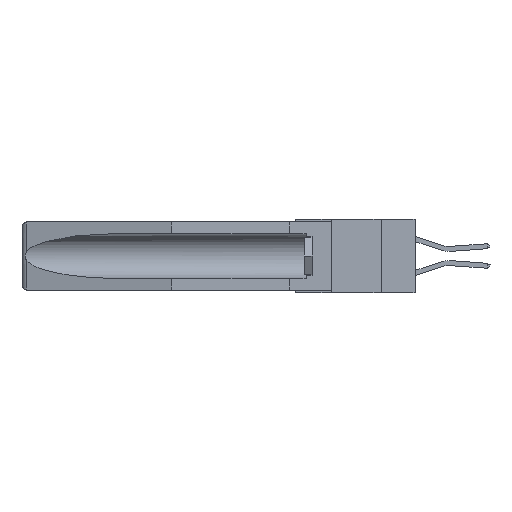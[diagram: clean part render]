
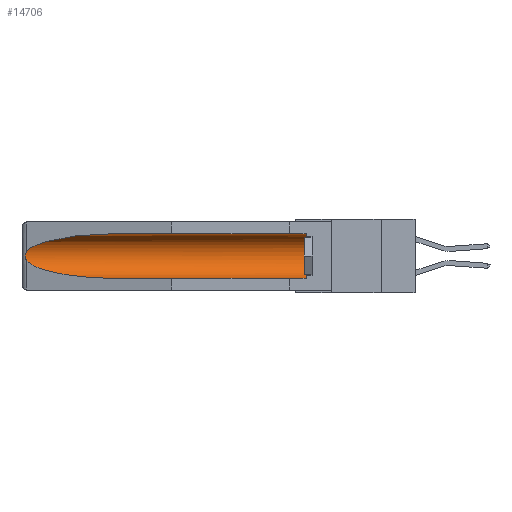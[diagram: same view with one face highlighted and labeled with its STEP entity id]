
A CAD part, left-side view. The second image highlights one B-rep face of the part: STEP entity #14706.
In plain terms, the highlighted cylindrical face has radius 2.857 mm (diameter 5.715 mm), a partial arc.
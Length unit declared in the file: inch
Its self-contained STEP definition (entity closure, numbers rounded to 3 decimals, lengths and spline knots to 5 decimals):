
#239 = DIRECTION ( 'NONE',  ( 0., 0., 1. ) ) ;
#935 = DIRECTION ( 'NONE',  ( 0., 1., 0. ) ) ;
#995 = VECTOR ( 'NONE', #17633, 39.37008 ) ;
#1039 = EDGE_CURVE ( 'NONE', #2040, #2214, #3369, .T. ) ;
#1953 = CARTESIAN_POINT ( 'NONE',  ( 0.26654, 1.53092, -0.15636 ) ) ;
#2040 = VERTEX_POINT ( 'NONE', #22768 ) ;
#2155 = CARTESIAN_POINT ( 'NONE',  ( 0.2673, 1.53269, -0.17917 ) ) ;
#2214 = VERTEX_POINT ( 'NONE', #13699 ) ;
#2488 = LINE ( 'NONE', #27379, #21067 ) ;
#3369 = B_SPLINE_CURVE_WITH_KNOTS ( 'NONE', 3,
 ( #18769, #9451, #1953, #23361, #26036, #16566, #2155, #11779, #23762, #25623 ),
 .UNSPECIFIED., .F., .F.,
 ( 4, 2, 2, 2, 4 ),
 ( 0., 0.00029, 0.00058, 0.00087, 0.00117 ),
 .UNSPECIFIED. ) ;
#3976 = VERTEX_POINT ( 'NONE', #26563 ) ;
#4784 = ORIENTED_EDGE ( 'NONE', *, *, #29915, .T. ) ;
#5179 = CARTESIAN_POINT ( 'NONE',  ( 0.21114, 1.30732, -0.059 ) ) ;
#5483 = CARTESIAN_POINT ( 'NONE',  ( 0.26537, 1.52718, -0.14972 ) ) ;
#5624 = AXIS2_PLACEMENT_3D ( 'NONE', #7690, #24319, #239 ) ;
#6420 = VERTEX_POINT ( 'NONE', #10971 ) ;
#7472 = CARTESIAN_POINT ( 'NONE',  ( 0.155, 1.07973, -0.059 ) ) ;
#7690 = CARTESIAN_POINT ( 'NONE',  ( 0.155, -0.30754, -0.1715 ) ) ;
#8312 = CARTESIAN_POINT ( 'NONE',  ( 0.155, -0.30754, -0.284 ) ) ;
#8531 = CARTESIAN_POINT ( 'NONE',  ( 0.26537, 1.52718, -0.19328 ) ) ;
#8636 = CARTESIAN_POINT ( 'NONE',  ( 0.21114, 1.30732, -0.284 ) ) ;
#9451 = CARTESIAN_POINT ( 'NONE',  ( 0.26597, 1.52961, -0.15275 ) ) ;
#9853 = ORIENTED_EDGE ( 'NONE', *, *, #19906, .F. ) ;
#9854 =( BOUNDED_CURVE ( )  B_SPLINE_CURVE ( 3, ( #8531, #11002, #8636, #13080 ),
 .UNSPECIFIED., .F., .F. ) 
 B_SPLINE_CURVE_WITH_KNOTS ( ( 4, 4 ),
 ( 0.1948, 1.5708 ),
 .UNSPECIFIED. ) 
 CURVE ( )  GEOMETRIC_REPRESENTATION_ITEM ( )  RATIONAL_B_SPLINE_CURVE ( ( 1., 0.848, 0.848, 1. ) ) 
 REPRESENTATION_ITEM ( '' )  );
#9869 = CARTESIAN_POINT ( 'NONE',  ( 0.155, 1.07973, -0.059 ) ) ;
#10153 = CIRCLE ( 'NONE', #29092, 0.1125 ) ;
#10298 = ORIENTED_EDGE ( 'NONE', *, *, #19920, .T. ) ;
#10971 = CARTESIAN_POINT ( 'NONE',  ( 0.155, 0.126, -0.284 ) ) ;
#11002 = CARTESIAN_POINT ( 'NONE',  ( 0.25451, 1.48313, -0.24835 ) ) ;
#11112 =( BOUNDED_CURVE ( )  B_SPLINE_CURVE ( 3, ( #9869, #5179, #24186, #5483 ),
 .UNSPECIFIED., .F., .F. ) 
 B_SPLINE_CURVE_WITH_KNOTS ( ( 4, 4 ),
 ( 4.71239, 6.08839 ),
 .UNSPECIFIED. ) 
 CURVE ( )  GEOMETRIC_REPRESENTATION_ITEM ( )  RATIONAL_B_SPLINE_CURVE ( ( 1., 0.848, 0.848, 1. ) ) 
 REPRESENTATION_ITEM ( '' )  );
#11709 = EDGE_CURVE ( 'NONE', #2214, #3976, #9854, .T. ) ;
#11779 = CARTESIAN_POINT ( 'NONE',  ( 0.26655, 1.53094, -0.18657 ) ) ;
#12750 = DIRECTION ( 'NONE',  ( 0., -1., 0. ) ) ;
#13080 = CARTESIAN_POINT ( 'NONE',  ( 0.155, 1.07973, -0.284 ) ) ;
#13699 = CARTESIAN_POINT ( 'NONE',  ( 0.26537, 1.52718, -0.19328 ) ) ;
#14258 = CARTESIAN_POINT ( 'NONE',  ( 0.155, 0.126, -0.059 ) ) ;
#14500 = VERTEX_POINT ( 'NONE', #14258 ) ;
#14706 = ADVANCED_FACE ( 'NONE', ( #22553 ), #16217, .F. ) ;
#15033 = EDGE_CURVE ( 'NONE', #19757, #2040, #11112, .T. ) ;
#16217 = CYLINDRICAL_SURFACE ( 'NONE', #5624, 0.1125 ) ;
#16566 = CARTESIAN_POINT ( 'NONE',  ( 0.2675, 1.53308, -0.17534 ) ) ;
#17633 = DIRECTION ( 'NONE',  ( 0., 1., 0. ) ) ;
#18769 = CARTESIAN_POINT ( 'NONE',  ( 0.26537, 1.52718, -0.14972 ) ) ;
#19604 = ORIENTED_EDGE ( 'NONE', *, *, #15033, .T. ) ;
#19730 = CARTESIAN_POINT ( 'NONE',  ( 0.155, 0.126, -0.1715 ) ) ;
#19757 = VERTEX_POINT ( 'NONE', #7472 ) ;
#19906 = EDGE_CURVE ( 'NONE', #6420, #3976, #28094, .T. ) ;
#19920 = EDGE_CURVE ( 'NONE', #14500, #19757, #2488, .T. ) ;
#21067 = VECTOR ( 'NONE', #935, 39.37008 ) ;
#22553 = FACE_OUTER_BOUND ( 'NONE', #26190, .T. ) ;
#22768 = CARTESIAN_POINT ( 'NONE',  ( 0.26537, 1.52718, -0.14972 ) ) ;
#23361 = CARTESIAN_POINT ( 'NONE',  ( 0.2673, 1.5327, -0.16383 ) ) ;
#23762 = CARTESIAN_POINT ( 'NONE',  ( 0.26597, 1.5296, -0.19026 ) ) ;
#24186 = CARTESIAN_POINT ( 'NONE',  ( 0.25451, 1.48313, -0.09465 ) ) ;
#24319 = DIRECTION ( 'NONE',  ( 0., 1., 0. ) ) ;
#25623 = CARTESIAN_POINT ( 'NONE',  ( 0.26537, 1.52718, -0.19328 ) ) ;
#26036 = CARTESIAN_POINT ( 'NONE',  ( 0.2675, 1.53308, -0.16763 ) ) ;
#26190 = EDGE_LOOP ( 'NONE', ( #19604, #27607, #28913, #9853, #4784, #10298 ) ) ;
#26563 = CARTESIAN_POINT ( 'NONE',  ( 0.155, 1.07973, -0.284 ) ) ;
#27379 = CARTESIAN_POINT ( 'NONE',  ( 0.155, -0.30754, -0.059 ) ) ;
#27607 = ORIENTED_EDGE ( 'NONE', *, *, #1039, .T. ) ;
#28094 = LINE ( 'NONE', #8312, #995 ) ;
#28913 = ORIENTED_EDGE ( 'NONE', *, *, #11709, .T. ) ;
#29092 = AXIS2_PLACEMENT_3D ( 'NONE', #19730, #12750, #29470 ) ;
#29470 = DIRECTION ( 'NONE',  ( 0., 0., 1. ) ) ;
#29915 = EDGE_CURVE ( 'NONE', #6420, #14500, #10153, .T. ) ;
